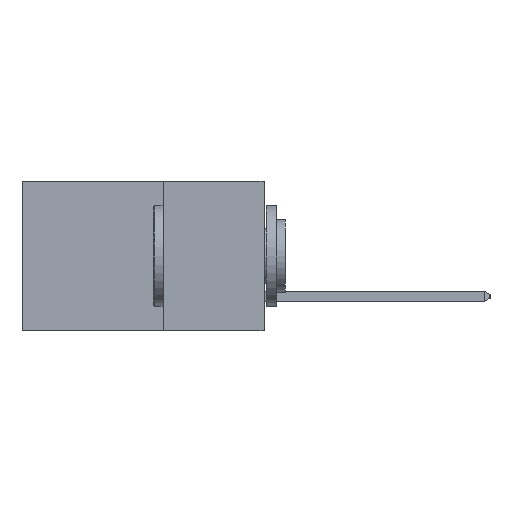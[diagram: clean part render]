
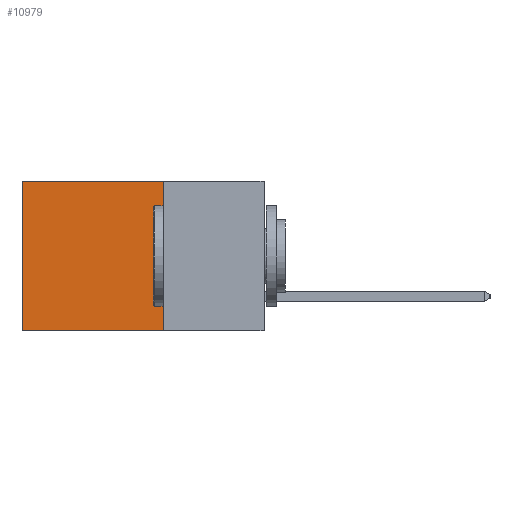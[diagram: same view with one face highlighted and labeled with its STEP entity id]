
A CAD part, left-side view. The second image highlights one B-rep face of the part: STEP entity #10979.
In plain terms, the highlighted planar face has unit normal (-1, 0, 0).
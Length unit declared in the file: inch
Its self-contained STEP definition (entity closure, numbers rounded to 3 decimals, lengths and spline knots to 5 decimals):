
#269 = EDGE_CURVE ( 'NONE', #9138, #13236, #12541, .T. ) ;
#273 = DIRECTION ( 'NONE',  ( 0., 0., -1. ) ) ;
#540 = ORIENTED_EDGE ( 'NONE', *, *, #12573, .T. ) ;
#737 = DIRECTION ( 'NONE',  ( 0., 0., -1. ) ) ;
#1309 = CARTESIAN_POINT ( 'NONE',  ( 0.2615, 0.6, -0.37 ) ) ;
#1830 = LINE ( 'NONE', #9861, #2741 ) ;
#1906 = CARTESIAN_POINT ( 'NONE',  ( 0.2615, 0.6, 0. ) ) ;
#2741 = VECTOR ( 'NONE', #9691, 39.37008 ) ;
#2777 = DIRECTION ( 'NONE',  ( 0., 0., -1. ) ) ;
#2852 = EDGE_CURVE ( 'NONE', #9138, #9761, #1830, .T. ) ;
#2956 = CARTESIAN_POINT ( 'NONE',  ( 0.2615, 0.25, -0.37 ) ) ;
#4440 = VECTOR ( 'NONE', #273, 39.37008 ) ;
#5060 = CARTESIAN_POINT ( 'NONE',  ( 0.2615, 0.25, -0.37 ) ) ;
#5251 = CARTESIAN_POINT ( 'NONE',  ( 0.2615, 0.25, -0.37 ) ) ;
#5919 = LINE ( 'NONE', #5251, #17425 ) ;
#8291 = CARTESIAN_POINT ( 'NONE',  ( 0.2615, 0.25, -0.37 ) ) ;
#8590 = VERTEX_POINT ( 'NONE', #17943 ) ;
#9138 = VERTEX_POINT ( 'NONE', #9656 ) ;
#9371 = DIRECTION ( 'NONE',  ( 1., 0., 0. ) ) ;
#9521 = LINE ( 'NONE', #1309, #9957 ) ;
#9656 = CARTESIAN_POINT ( 'NONE',  ( 0.2615, 0.25, 0. ) ) ;
#9691 = DIRECTION ( 'NONE',  ( 0., 1., 0. ) ) ;
#9761 = VERTEX_POINT ( 'NONE', #1906 ) ;
#9861 = CARTESIAN_POINT ( 'NONE',  ( 0.2615, 0.25, 0. ) ) ;
#9957 = VECTOR ( 'NONE', #2777, 39.37008 ) ;
#10848 = AXIS2_PLACEMENT_3D ( 'NONE', #5060, #9371, #737 ) ;
#10979 = ADVANCED_FACE ( 'NONE', ( #11152 ), #17978, .F. ) ;
#11152 = FACE_OUTER_BOUND ( 'NONE', #14520, .T. ) ;
#12323 = EDGE_CURVE ( 'NONE', #13236, #8590, #5919, .T. ) ;
#12541 = LINE ( 'NONE', #2956, #4440 ) ;
#12573 = EDGE_CURVE ( 'NONE', #9761, #8590, #9521, .T. ) ;
#13236 = VERTEX_POINT ( 'NONE', #8291 ) ;
#13626 = ORIENTED_EDGE ( 'NONE', *, *, #12323, .F. ) ;
#14520 = EDGE_LOOP ( 'NONE', ( #540, #13626, #17107, #15984 ) ) ;
#15346 = DIRECTION ( 'NONE',  ( 0., 1., 0. ) ) ;
#15984 = ORIENTED_EDGE ( 'NONE', *, *, #2852, .T. ) ;
#17107 = ORIENTED_EDGE ( 'NONE', *, *, #269, .F. ) ;
#17425 = VECTOR ( 'NONE', #15346, 39.37008 ) ;
#17943 = CARTESIAN_POINT ( 'NONE',  ( 0.2615, 0.6, -0.37 ) ) ;
#17978 = PLANE ( 'NONE',  #10848 ) ;
